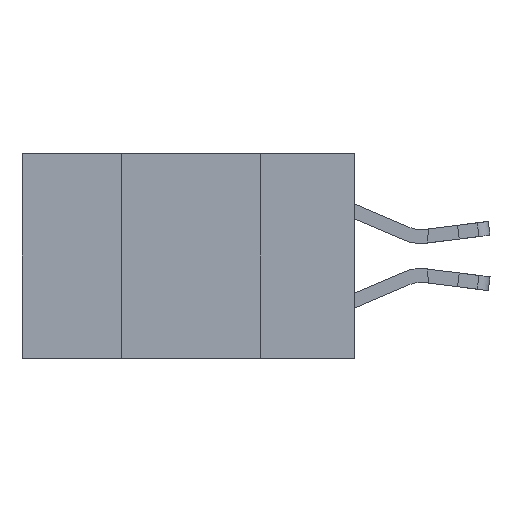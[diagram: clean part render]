
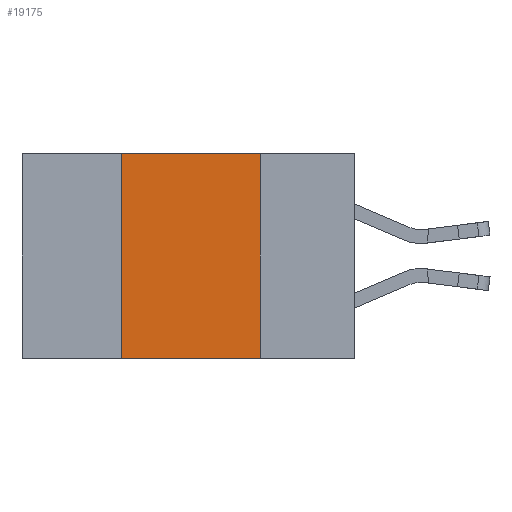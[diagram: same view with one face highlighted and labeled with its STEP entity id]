
A CAD part, left-side view. The second image highlights one B-rep face of the part: STEP entity #19175.
In plain terms, the highlighted planar face has unit normal (-1, 0, 0).
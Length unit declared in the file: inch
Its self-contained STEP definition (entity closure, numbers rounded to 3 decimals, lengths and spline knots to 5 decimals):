
#50 = CARTESIAN_POINT ( 'NONE',  ( 0., 0.17, 0. ) ) ;
#352 = VERTEX_POINT ( 'NONE', #5609 ) ;
#2683 = EDGE_CURVE ( 'NONE', #18057, #14291, #4762, .T. ) ;
#2706 = ORIENTED_EDGE ( 'NONE', *, *, #19045, .T. ) ;
#3827 = LINE ( 'NONE', #19982, #21668 ) ;
#4300 = VERTEX_POINT ( 'NONE', #19555 ) ;
#4700 = AXIS2_PLACEMENT_3D ( 'NONE', #20244, #21857, #12059 ) ;
#4762 = LINE ( 'NONE', #8882, #6727 ) ;
#5012 = FACE_OUTER_BOUND ( 'NONE', #12235, .T. ) ;
#5609 = CARTESIAN_POINT ( 'NONE',  ( 0., 0.42, -0.37 ) ) ;
#6341 = ORIENTED_EDGE ( 'NONE', *, *, #2683, .F. ) ;
#6638 = DIRECTION ( 'NONE',  ( 0., -1., 0. ) ) ;
#6727 = VECTOR ( 'NONE', #10574, 39.37008 ) ;
#7779 = LINE ( 'NONE', #16693, #12756 ) ;
#7959 = DIRECTION ( 'NONE',  ( 0., -1., 0. ) ) ;
#8882 = CARTESIAN_POINT ( 'NONE',  ( 0., 0.17, 0. ) ) ;
#10574 = DIRECTION ( 'NONE',  ( 0., 0., -1. ) ) ;
#10896 = ORIENTED_EDGE ( 'NONE', *, *, #17821, .F. ) ;
#12059 = DIRECTION ( 'NONE',  ( 0., 0., -1. ) ) ;
#12235 = EDGE_LOOP ( 'NONE', ( #6341, #10896, #15798, #2706 ) ) ;
#12756 = VECTOR ( 'NONE', #6638, 39.37008 ) ;
#13426 = DIRECTION ( 'NONE',  ( 0., 0., 1. ) ) ;
#14270 = VECTOR ( 'NONE', #7959, 39.37008 ) ;
#14291 = VERTEX_POINT ( 'NONE', #19668 ) ;
#14799 = LINE ( 'NONE', #19563, #14270 ) ;
#15798 = ORIENTED_EDGE ( 'NONE', *, *, #20118, .F. ) ;
#16693 = CARTESIAN_POINT ( 'NONE',  ( 0., 0.6, -0.37 ) ) ;
#16979 = PLANE ( 'NONE',  #4700 ) ;
#17821 = EDGE_CURVE ( 'NONE', #4300, #18057, #14799, .T. ) ;
#18057 = VERTEX_POINT ( 'NONE', #50 ) ;
#19045 = EDGE_CURVE ( 'NONE', #352, #14291, #7779, .T. ) ;
#19175 = ADVANCED_FACE ( 'NONE', ( #5012 ), #16979, .F. ) ;
#19555 = CARTESIAN_POINT ( 'NONE',  ( 0., 0.42, 0. ) ) ;
#19563 = CARTESIAN_POINT ( 'NONE',  ( 0., 0.6, 0. ) ) ;
#19668 = CARTESIAN_POINT ( 'NONE',  ( 0., 0.17, -0.37 ) ) ;
#19982 = CARTESIAN_POINT ( 'NONE',  ( 0., 0.42, 0. ) ) ;
#20118 = EDGE_CURVE ( 'NONE', #352, #4300, #3827, .T. ) ;
#20244 = CARTESIAN_POINT ( 'NONE',  ( 0., 0.6, 0. ) ) ;
#21668 = VECTOR ( 'NONE', #13426, 39.37008 ) ;
#21857 = DIRECTION ( 'NONE',  ( 1., 0., 0. ) ) ;
